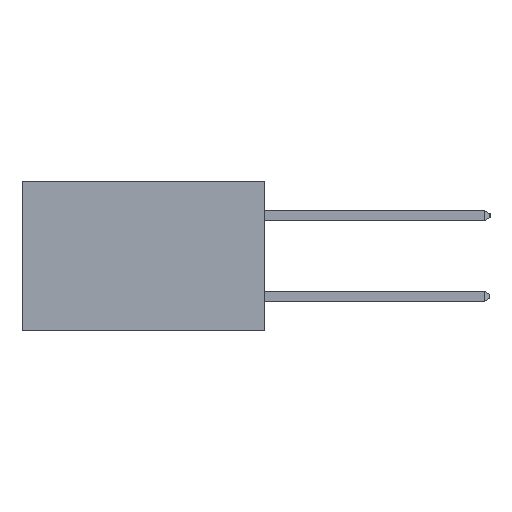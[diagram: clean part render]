
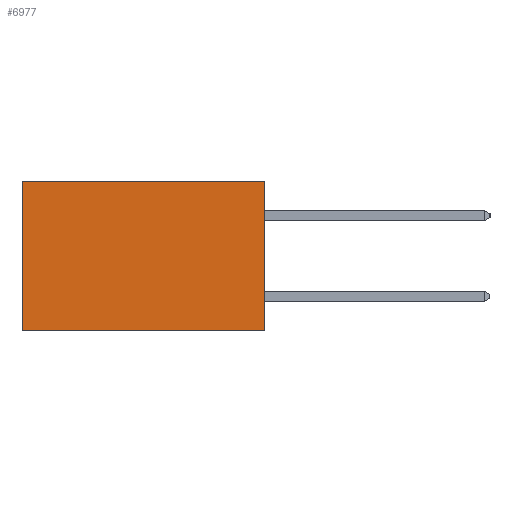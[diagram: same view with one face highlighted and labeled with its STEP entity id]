
A CAD part, left-side view. The second image highlights one B-rep face of the part: STEP entity #6977.
In plain terms, the highlighted planar face has unit normal (-1, 0, 0).
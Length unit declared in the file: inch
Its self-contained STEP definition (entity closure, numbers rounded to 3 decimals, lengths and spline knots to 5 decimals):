
#1230 = VERTEX_POINT ( 'NONE', #8619 ) ;
#1718 = ORIENTED_EDGE ( 'NONE', *, *, #2790, .F. ) ;
#1908 = CARTESIAN_POINT ( 'NONE',  ( 0.298, 0., 0. ) ) ;
#2790 = EDGE_CURVE ( 'NONE', #3099, #1230, #3797, .T. ) ;
#3099 = VERTEX_POINT ( 'NONE', #1908 ) ;
#3797 = LINE ( 'NONE', #5245, #24835 ) ;
#4110 = ORIENTED_EDGE ( 'NONE', *, *, #11855, .F. ) ;
#4769 = CARTESIAN_POINT ( 'NONE',  ( 0.298, 0.6, 0. ) ) ;
#5245 = CARTESIAN_POINT ( 'NONE',  ( 0.298, 0., 0. ) ) ;
#5362 = DIRECTION ( 'NONE',  ( 0., 1., 0. ) ) ;
#6156 = PLANE ( 'NONE',  #7524 ) ;
#6977 = ADVANCED_FACE ( 'NONE', ( #18427 ), #6156, .F. ) ;
#7027 = DIRECTION ( 'NONE',  ( 0., 1., 0. ) ) ;
#7524 = AXIS2_PLACEMENT_3D ( 'NONE', #7638, #7841, #7806 ) ;
#7638 = CARTESIAN_POINT ( 'NONE',  ( 0.298, 0., 0. ) ) ;
#7806 = DIRECTION ( 'NONE',  ( 0., 0., -1. ) ) ;
#7807 = LINE ( 'NONE', #4769, #11895 ) ;
#7819 = DIRECTION ( 'NONE',  ( 0., 0., -1. ) ) ;
#7841 = DIRECTION ( 'NONE',  ( 1., 0., 0. ) ) ;
#8619 = CARTESIAN_POINT ( 'NONE',  ( 0.298, 0., -0.37 ) ) ;
#9204 = LINE ( 'NONE', #13084, #13910 ) ;
#11848 = VECTOR ( 'NONE', #5362, 39.37008 ) ;
#11855 = EDGE_CURVE ( 'NONE', #1230, #21929, #17298, .T. ) ;
#11895 = VECTOR ( 'NONE', #18965, 39.37008 ) ;
#13084 = CARTESIAN_POINT ( 'NONE',  ( 0.298, 0., 0. ) ) ;
#13910 = VECTOR ( 'NONE', #7027, 39.37008 ) ;
#16991 = EDGE_LOOP ( 'NONE', ( #23339, #4110, #1718, #17542 ) ) ;
#17298 = LINE ( 'NONE', #21543, #11848 ) ;
#17542 = ORIENTED_EDGE ( 'NONE', *, *, #24784, .T. ) ;
#18427 = FACE_OUTER_BOUND ( 'NONE', #16991, .T. ) ;
#18965 = DIRECTION ( 'NONE',  ( 0., 0., -1. ) ) ;
#19534 = EDGE_CURVE ( 'NONE', #26409, #21929, #7807, .T. ) ;
#20514 = CARTESIAN_POINT ( 'NONE',  ( 0.298, 0.6, -0.37 ) ) ;
#21543 = CARTESIAN_POINT ( 'NONE',  ( 0.298, 0., -0.37 ) ) ;
#21929 = VERTEX_POINT ( 'NONE', #20514 ) ;
#23339 = ORIENTED_EDGE ( 'NONE', *, *, #19534, .T. ) ;
#24449 = CARTESIAN_POINT ( 'NONE',  ( 0.298, 0.6, 0. ) ) ;
#24784 = EDGE_CURVE ( 'NONE', #3099, #26409, #9204, .T. ) ;
#24835 = VECTOR ( 'NONE', #7819, 39.37008 ) ;
#26409 = VERTEX_POINT ( 'NONE', #24449 ) ;
